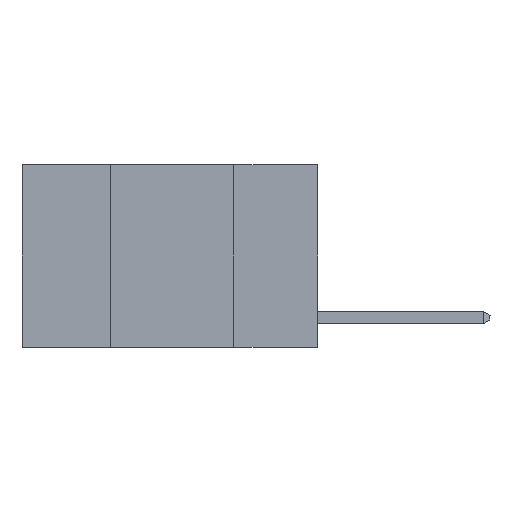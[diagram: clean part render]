
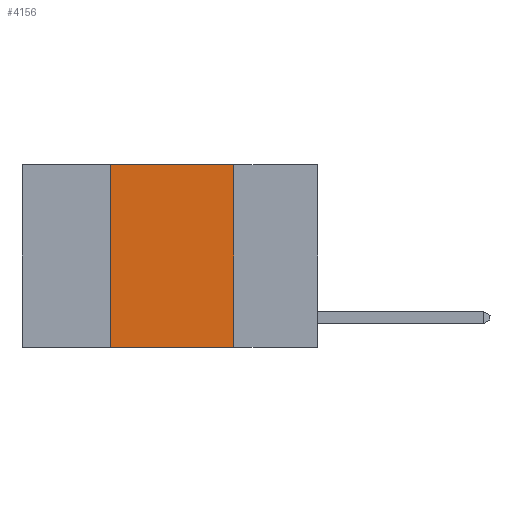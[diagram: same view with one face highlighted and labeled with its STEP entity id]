
A CAD part, left-side view. The second image highlights one B-rep face of the part: STEP entity #4156.
In plain terms, the highlighted planar face has unit normal (-1, 0, 0).
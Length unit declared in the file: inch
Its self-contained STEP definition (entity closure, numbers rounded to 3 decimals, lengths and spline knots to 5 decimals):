
#247 = LINE ( 'NONE', #1419, #20893 ) ;
#1146 = CARTESIAN_POINT ( 'NONE',  ( 0., 0.42, 0. ) ) ;
#1305 = CARTESIAN_POINT ( 'NONE',  ( 0., 0.6, 0. ) ) ;
#1363 = PLANE ( 'NONE',  #18027 ) ;
#1419 = CARTESIAN_POINT ( 'NONE',  ( 0., 0.17, 0. ) ) ;
#3345 = CARTESIAN_POINT ( 'NONE',  ( 0., 0.17, -0.37 ) ) ;
#3858 = DIRECTION ( 'NONE',  ( 0., 0., 1. ) ) ;
#3990 = ORIENTED_EDGE ( 'NONE', *, *, #8093, .F. ) ;
#4156 = ADVANCED_FACE ( 'NONE', ( #10797 ), #1363, .F. ) ;
#4329 = CARTESIAN_POINT ( 'NONE',  ( 0., 0.6, -0.37 ) ) ;
#8093 = EDGE_CURVE ( 'NONE', #13321, #20759, #247, .T. ) ;
#10213 = LINE ( 'NONE', #23822, #20784 ) ;
#10338 = DIRECTION ( 'NONE',  ( 0., -1., 0. ) ) ;
#10797 = FACE_OUTER_BOUND ( 'NONE', #16233, .T. ) ;
#11935 = CARTESIAN_POINT ( 'NONE',  ( 0., 0.42, -0.37 ) ) ;
#11942 = DIRECTION ( 'NONE',  ( 0., -1., 0. ) ) ;
#12269 = VECTOR ( 'NONE', #10338, 39.37008 ) ;
#13092 = LINE ( 'NONE', #13754, #17159 ) ;
#13321 = VERTEX_POINT ( 'NONE', #18831 ) ;
#13754 = CARTESIAN_POINT ( 'NONE',  ( 0., 0.42, 0. ) ) ;
#15860 = DIRECTION ( 'NONE',  ( 1., 0., 0. ) ) ;
#16233 = EDGE_LOOP ( 'NONE', ( #3990, #19856, #25057, #21130 ) ) ;
#17159 = VECTOR ( 'NONE', #3858, 39.37008 ) ;
#17987 = EDGE_CURVE ( 'NONE', #18510, #20759, #22845, .T. ) ;
#18027 = AXIS2_PLACEMENT_3D ( 'NONE', #1305, #15860, #24396 ) ;
#18510 = VERTEX_POINT ( 'NONE', #11935 ) ;
#18831 = CARTESIAN_POINT ( 'NONE',  ( 0., 0.17, 0. ) ) ;
#19546 = EDGE_CURVE ( 'NONE', #18510, #20067, #13092, .T. ) ;
#19856 = ORIENTED_EDGE ( 'NONE', *, *, #24571, .F. ) ;
#20067 = VERTEX_POINT ( 'NONE', #1146 ) ;
#20759 = VERTEX_POINT ( 'NONE', #3345 ) ;
#20784 = VECTOR ( 'NONE', #11942, 39.37008 ) ;
#20893 = VECTOR ( 'NONE', #21422, 39.37008 ) ;
#21130 = ORIENTED_EDGE ( 'NONE', *, *, #17987, .T. ) ;
#21422 = DIRECTION ( 'NONE',  ( 0., 0., -1. ) ) ;
#22845 = LINE ( 'NONE', #4329, #12269 ) ;
#23822 = CARTESIAN_POINT ( 'NONE',  ( 0., 0.6, 0. ) ) ;
#24396 = DIRECTION ( 'NONE',  ( 0., 0., -1. ) ) ;
#24571 = EDGE_CURVE ( 'NONE', #20067, #13321, #10213, .T. ) ;
#25057 = ORIENTED_EDGE ( 'NONE', *, *, #19546, .F. ) ;
